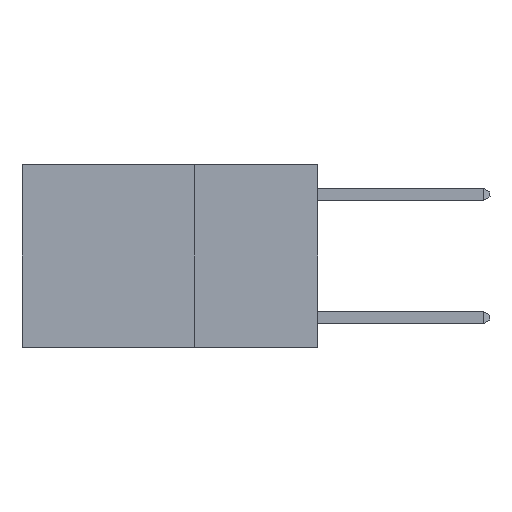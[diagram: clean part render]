
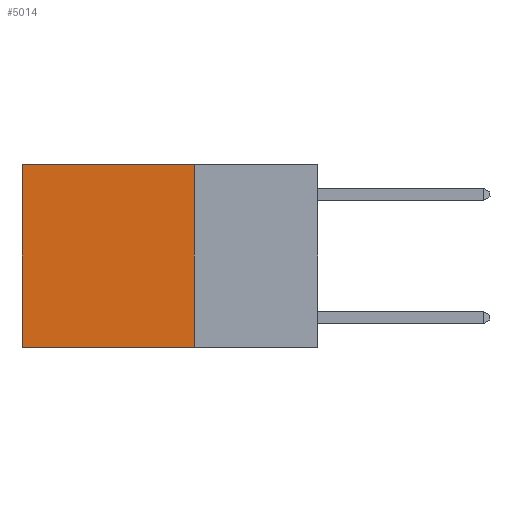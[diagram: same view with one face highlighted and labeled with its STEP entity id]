
A CAD part, left-side view. The second image highlights one B-rep face of the part: STEP entity #5014.
In plain terms, the highlighted planar face has unit normal (-1, 0, 0).
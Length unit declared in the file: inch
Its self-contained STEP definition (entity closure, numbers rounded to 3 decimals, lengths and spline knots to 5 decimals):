
#82 = LINE ( 'NONE', #2771, #2344 ) ;
#318 = LINE ( 'NONE', #1716, #8627 ) ;
#759 = CARTESIAN_POINT ( 'NONE',  ( 0.2625, 0.25, 0. ) ) ;
#830 = DIRECTION ( 'NONE',  ( 0., 1., 0. ) ) ;
#1135 = LINE ( 'NONE', #3401, #2808 ) ;
#1289 = EDGE_CURVE ( 'NONE', #2092, #5260, #318, .T. ) ;
#1357 = AXIS2_PLACEMENT_3D ( 'NONE', #759, #8477, #2402 ) ;
#1540 = ORIENTED_EDGE ( 'NONE', *, *, #1289, .T. ) ;
#1716 = CARTESIAN_POINT ( 'NONE',  ( 0.2625, 0.25, 0. ) ) ;
#2092 = VERTEX_POINT ( 'NONE', #3605 ) ;
#2324 = EDGE_CURVE ( 'NONE', #2092, #5964, #1135, .T. ) ;
#2344 = VECTOR ( 'NONE', #2823, 39.37008 ) ;
#2402 = DIRECTION ( 'NONE',  ( 0., 0., -1. ) ) ;
#2405 = DIRECTION ( 'NONE',  ( 0., 1., 0. ) ) ;
#2771 = CARTESIAN_POINT ( 'NONE',  ( 0.2625, 0.6, 0. ) ) ;
#2808 = VECTOR ( 'NONE', #5499, 39.37008 ) ;
#2823 = DIRECTION ( 'NONE',  ( 0., 0., -1. ) ) ;
#3065 = PLANE ( 'NONE',  #1357 ) ;
#3281 = EDGE_CURVE ( 'NONE', #5964, #7530, #6198, .T. ) ;
#3323 = EDGE_LOOP ( 'NONE', ( #6049, #3886, #4556, #1540 ) ) ;
#3401 = CARTESIAN_POINT ( 'NONE',  ( 0.2625, 0.25, 0. ) ) ;
#3605 = CARTESIAN_POINT ( 'NONE',  ( 0.2625, 0.25, 0. ) ) ;
#3660 = EDGE_CURVE ( 'NONE', #5260, #7530, #82, .T. ) ;
#3729 = CARTESIAN_POINT ( 'NONE',  ( 0.2625, 0.6, -0.37 ) ) ;
#3886 = ORIENTED_EDGE ( 'NONE', *, *, #3281, .F. ) ;
#4554 = CARTESIAN_POINT ( 'NONE',  ( 0.2625, 0.25, -0.37 ) ) ;
#4556 = ORIENTED_EDGE ( 'NONE', *, *, #2324, .F. ) ;
#5014 = ADVANCED_FACE ( 'NONE', ( #7549 ), #3065, .F. ) ;
#5260 = VERTEX_POINT ( 'NONE', #5473 ) ;
#5473 = CARTESIAN_POINT ( 'NONE',  ( 0.2625, 0.6, 0. ) ) ;
#5499 = DIRECTION ( 'NONE',  ( 0., 0., -1. ) ) ;
#5964 = VERTEX_POINT ( 'NONE', #4554 ) ;
#6049 = ORIENTED_EDGE ( 'NONE', *, *, #3660, .T. ) ;
#6198 = LINE ( 'NONE', #6940, #8146 ) ;
#6940 = CARTESIAN_POINT ( 'NONE',  ( 0.2625, 0.25, -0.37 ) ) ;
#7530 = VERTEX_POINT ( 'NONE', #3729 ) ;
#7549 = FACE_OUTER_BOUND ( 'NONE', #3323, .T. ) ;
#8146 = VECTOR ( 'NONE', #830, 39.37008 ) ;
#8477 = DIRECTION ( 'NONE',  ( 1., 0., 0. ) ) ;
#8627 = VECTOR ( 'NONE', #2405, 39.37008 ) ;
